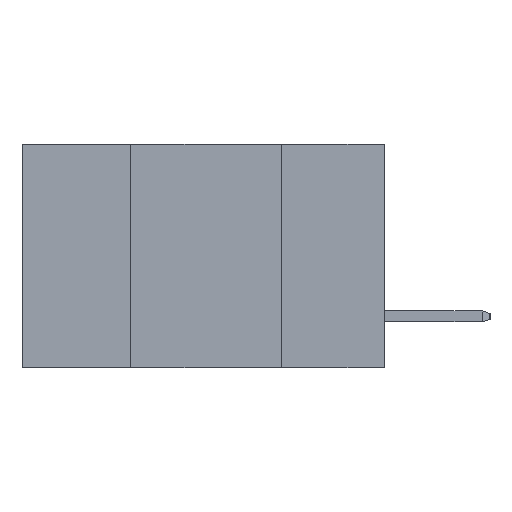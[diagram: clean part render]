
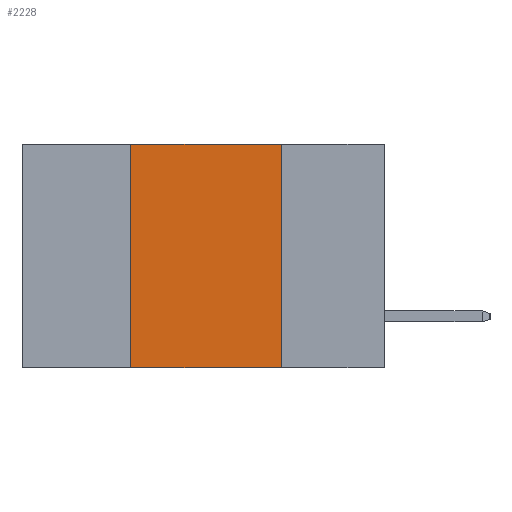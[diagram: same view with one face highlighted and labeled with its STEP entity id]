
A CAD part, left-side view. The second image highlights one B-rep face of the part: STEP entity #2228.
In plain terms, the highlighted planar face has unit normal (-1, 0, 0).
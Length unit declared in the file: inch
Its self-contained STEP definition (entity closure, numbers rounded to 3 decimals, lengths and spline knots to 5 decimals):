
#237 = EDGE_LOOP ( 'NONE', ( #1581, #4567, #2334, #1849 ) ) ;
#491 = VERTEX_POINT ( 'NONE', #9417 ) ;
#566 = VECTOR ( 'NONE', #6908, 39.37008 ) ;
#807 = VERTEX_POINT ( 'NONE', #3709 ) ;
#960 = DIRECTION ( 'NONE',  ( 0., 0., 1. ) ) ;
#1581 = ORIENTED_EDGE ( 'NONE', *, *, #8256, .F. ) ;
#1849 = ORIENTED_EDGE ( 'NONE', *, *, #7261, .T. ) ;
#2180 = DIRECTION ( 'NONE',  ( 0., -1., 0. ) ) ;
#2215 = CARTESIAN_POINT ( 'NONE',  ( 0., 0.42, -0.37 ) ) ;
#2228 = ADVANCED_FACE ( 'NONE', ( #3941 ), #6402, .F. ) ;
#2334 = ORIENTED_EDGE ( 'NONE', *, *, #7028, .F. ) ;
#2653 = LINE ( 'NONE', #6165, #566 ) ;
#2934 = CARTESIAN_POINT ( 'NONE',  ( 0., 0.6, -0.37 ) ) ;
#2984 = CARTESIAN_POINT ( 'NONE',  ( 0., 0.42, 0. ) ) ;
#3681 = LINE ( 'NONE', #4082, #9344 ) ;
#3709 = CARTESIAN_POINT ( 'NONE',  ( 0., 0.17, 0. ) ) ;
#3735 = VECTOR ( 'NONE', #960, 39.37008 ) ;
#3941 = FACE_OUTER_BOUND ( 'NONE', #237, .T. ) ;
#3992 = AXIS2_PLACEMENT_3D ( 'NONE', #7629, #8571, #5050 ) ;
#4082 = CARTESIAN_POINT ( 'NONE',  ( 0., 0.6, 0. ) ) ;
#4109 = VERTEX_POINT ( 'NONE', #2984 ) ;
#4567 = ORIENTED_EDGE ( 'NONE', *, *, #9632, .F. ) ;
#4829 = DIRECTION ( 'NONE',  ( 0., -1., 0. ) ) ;
#5050 = DIRECTION ( 'NONE',  ( 0., 0., -1. ) ) ;
#5552 = CARTESIAN_POINT ( 'NONE',  ( 0., 0.42, -0.37 ) ) ;
#5764 = LINE ( 'NONE', #5552, #3735 ) ;
#5874 = LINE ( 'NONE', #2934, #7615 ) ;
#6165 = CARTESIAN_POINT ( 'NONE',  ( 0., 0.17, -0.37 ) ) ;
#6402 = PLANE ( 'NONE',  #3992 ) ;
#6808 = VERTEX_POINT ( 'NONE', #2215 ) ;
#6908 = DIRECTION ( 'NONE',  ( 0., 0., -1. ) ) ;
#7028 = EDGE_CURVE ( 'NONE', #6808, #4109, #5764, .T. ) ;
#7261 = EDGE_CURVE ( 'NONE', #6808, #491, #5874, .T. ) ;
#7615 = VECTOR ( 'NONE', #2180, 39.37008 ) ;
#7629 = CARTESIAN_POINT ( 'NONE',  ( 0., 0.6, 0. ) ) ;
#8256 = EDGE_CURVE ( 'NONE', #807, #491, #2653, .T. ) ;
#8571 = DIRECTION ( 'NONE',  ( 1., 0., 0. ) ) ;
#9344 = VECTOR ( 'NONE', #4829, 39.37008 ) ;
#9417 = CARTESIAN_POINT ( 'NONE',  ( 0., 0.17, -0.37 ) ) ;
#9632 = EDGE_CURVE ( 'NONE', #4109, #807, #3681, .T. ) ;
